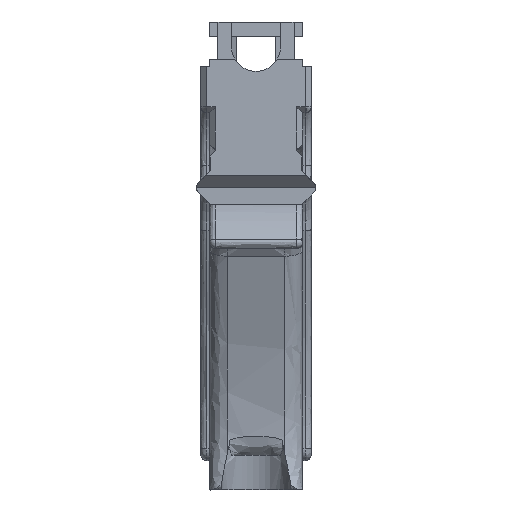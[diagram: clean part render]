
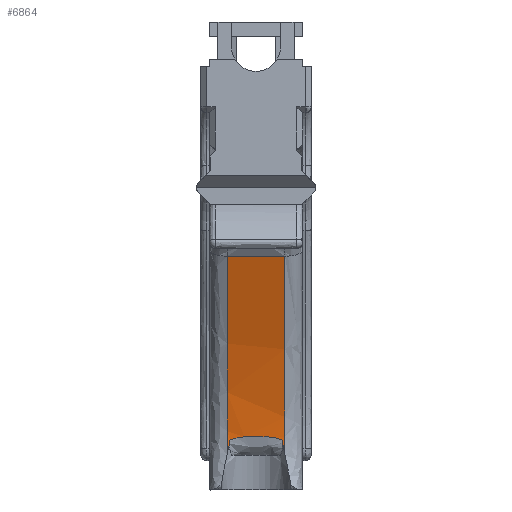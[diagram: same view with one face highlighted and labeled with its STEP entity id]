
A CAD part, front view. The second image highlights one B-rep face of the part: STEP entity #6864.
In plain terms, the highlighted free-form (B-spline) face has degree [5, 1] with [25, 2] control points.
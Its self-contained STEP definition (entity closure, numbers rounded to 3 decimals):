
#20=(
BOUNDED_SURFACE()
B_SPLINE_SURFACE(5,1,((#10581,#10582),(#10583,#10584),(#10585,#10586),(#10587,
#10588),(#10589,#10590),(#10591,#10592),(#10593,#10594),(#10595,#10596),
(#10597,#10598),(#10599,#10600),(#10601,#10602),(#10603,#10604),(#10605,
#10606),(#10607,#10608),(#10609,#10610),(#10611,#10612),(#10613,#10614),
(#10615,#10616),(#10617,#10618),(#10619,#10620),(#10621,#10622),(#10623,
#10624),(#10625,#10626),(#10627,#10628),(#10629,#10630)),.UNSPECIFIED.,
 .F.,.F.,.F.)
B_SPLINE_SURFACE_WITH_KNOTS((6,5,1,1,1,1,1,1,1,1,1,5,6),(2,2),(-1.404,
0.,0.1,0.2,0.3,0.4,0.5,0.6,0.7,0.8,0.9,1.,1.483),(-0.318,
1.908),.UNSPECIFIED.)
GEOMETRIC_REPRESENTATION_ITEM()
RATIONAL_B_SPLINE_SURFACE(((1.,1.),(1.,1.),(1.,1.),(1.,1.),(1.,1.),(1.,
1.),(1.,1.),(1.,1.),(1.,1.),(1.,1.),(1.,1.),(1.,1.),(1.,1.),(1.,1.),(1.,
1.),(1.,1.),(1.,1.),(1.,1.),(1.,1.),(1.,1.),(1.,1.),(1.,1.),(1.,1.),(1.,
1.),(1.,1.)))
REPRESENTATION_ITEM('')
SURFACE()
);
#200=B_SPLINE_CURVE_WITH_KNOTS('',3,(#10518,#10519,#10520,#10521,#10522,
#10523,#10524,#10525,#10526),.UNSPECIFIED.,.F.,.F.,(4,1,1,1,1,1,4),(-0.959,
-0.877,-0.755,-0.632,-0.386,
-0.141,-0.059),.UNSPECIFIED.);
#202=B_SPLINE_CURVE_WITH_KNOTS('',3,(#10632,#10633,#10634,#10635),
 .UNSPECIFIED.,.F.,.F.,(4,4),(-0.911,-0.711),
 .UNSPECIFIED.);
#203=B_SPLINE_CURVE_WITH_KNOTS('',3,(#10637,#10638,#10639,#10640,#10641,
#10642,#10643),.UNSPECIFIED.,.F.,.F.,(4,1,1,1,4),(-4.241,-2.995,
-1.749,-1.126,-0.582),.UNSPECIFIED.);
#204=B_SPLINE_CURVE_WITH_KNOTS('',3,(#10645,#10646,#10647,#10648),
 .UNSPECIFIED.,.F.,.F.,(4,4),(-1.29,-0.3),
 .UNSPECIFIED.);
#205=B_SPLINE_CURVE_WITH_KNOTS('',3,(#10650,#10651,#10652,#10653,#10654,
#10655,#10656),.UNSPECIFIED.,.F.,.F.,(4,1,1,1,4),(0.582,1.126,
1.749,2.995,4.241),.UNSPECIFIED.);
#206=B_SPLINE_CURVE_WITH_KNOTS('',3,(#10657,#10658,#10659,#10660),
 .UNSPECIFIED.,.F.,.F.,(4,4),(-0.243,0.),.UNSPECIFIED.);
#616=FACE_OUTER_BOUND('',#1000,.T.);
#1000=EDGE_LOOP('',(#4863,#4864,#4865,#4866,#4867,#4868));
#3012=VERTEX_POINT('',#10463);
#3014=VERTEX_POINT('',#10517);
#3016=VERTEX_POINT('',#10631);
#3017=VERTEX_POINT('',#10636);
#3018=VERTEX_POINT('',#10644);
#3019=VERTEX_POINT('',#10649);
#3720=EDGE_CURVE('',#3012,#3014,#200,.T.);
#3723=EDGE_CURVE('',#3016,#3012,#202,.T.);
#3724=EDGE_CURVE('',#3017,#3016,#203,.T.);
#3725=EDGE_CURVE('',#3018,#3017,#204,.T.);
#3726=EDGE_CURVE('',#3019,#3018,#205,.T.);
#3727=EDGE_CURVE('',#3014,#3019,#206,.T.);
#4863=ORIENTED_EDGE('',*,*,#3723,.F.);
#4864=ORIENTED_EDGE('',*,*,#3724,.F.);
#4865=ORIENTED_EDGE('',*,*,#3725,.F.);
#4866=ORIENTED_EDGE('',*,*,#3726,.F.);
#4867=ORIENTED_EDGE('',*,*,#3727,.F.);
#4868=ORIENTED_EDGE('',*,*,#3720,.F.);
#6864=ADVANCED_FACE('',(#616),#20,.F.);
#10463=CARTESIAN_POINT('',(12.379,-27.933,-61.535));
#10517=CARTESIAN_POINT('',(3.521,-27.933,-61.535));
#10518=CARTESIAN_POINT('Ctrl Pts',(12.379,-27.933,-61.535));
#10519=CARTESIAN_POINT('Ctrl Pts',(12.129,-27.934,-61.435));
#10520=CARTESIAN_POINT('Ctrl Pts',(11.484,-27.939,-61.226));
#10521=CARTESIAN_POINT('Ctrl Pts',(10.413,-27.946,-61.033));
#10522=CARTESIAN_POINT('Ctrl Pts',(8.771,-27.95,-60.907));
#10523=CARTESIAN_POINT('Ctrl Pts',(6.718,-27.951,-60.907));
#10524=CARTESIAN_POINT('Ctrl Pts',(4.803,-27.942,-61.102));
#10525=CARTESIAN_POINT('Ctrl Pts',(3.77,-27.934,-61.435));
#10526=CARTESIAN_POINT('Ctrl Pts',(3.521,-27.933,-61.535));
#10581=CARTESIAN_POINT('Ctrl Pts',(-3.18,-48.861,
-96.18));
#10582=CARTESIAN_POINT('Ctrl Pts',(19.08,-48.861,-96.18));
#10583=CARTESIAN_POINT('Ctrl Pts',(-3.18,-45.092,
-90.944));
#10584=CARTESIAN_POINT('Ctrl Pts',(19.08,-45.092,-90.944));
#10585=CARTESIAN_POINT('Ctrl Pts',(-3.18,-41.323,
-85.709));
#10586=CARTESIAN_POINT('Ctrl Pts',(19.08,-41.323,-85.709));
#10587=CARTESIAN_POINT('Ctrl Pts',(-3.18,-37.554,
-80.474));
#10588=CARTESIAN_POINT('Ctrl Pts',(19.08,-37.554,-80.474));
#10589=CARTESIAN_POINT('Ctrl Pts',(-3.18,-33.785,
-75.238));
#10590=CARTESIAN_POINT('Ctrl Pts',(19.08,-33.785,-75.238));
#10591=CARTESIAN_POINT('Ctrl Pts',(-3.18,-30.016,
-70.003));
#10592=CARTESIAN_POINT('Ctrl Pts',(19.08,-30.016,-70.003));
#10593=CARTESIAN_POINT('Ctrl Pts',(-3.18,-29.748,
-69.63));
#10594=CARTESIAN_POINT('Ctrl Pts',(19.08,-29.748,-69.63));
#10595=CARTESIAN_POINT('Ctrl Pts',(-3.18,-29.253,
-68.836));
#10596=CARTESIAN_POINT('Ctrl Pts',(19.08,-29.253,-68.836));
#10597=CARTESIAN_POINT('Ctrl Pts',(-3.18,-28.637,
-67.498));
#10598=CARTESIAN_POINT('Ctrl Pts',(19.08,-28.637,-67.498));
#10599=CARTESIAN_POINT('Ctrl Pts',(-3.18,-28.071,
-65.416));
#10600=CARTESIAN_POINT('Ctrl Pts',(19.08,-28.071,-65.416));
#10601=CARTESIAN_POINT('Ctrl Pts',(-3.18,-27.812,
-62.291));
#10602=CARTESIAN_POINT('Ctrl Pts',(19.08,-27.812,-62.291));
#10603=CARTESIAN_POINT('Ctrl Pts',(-3.18,-28.022,
-58.621));
#10604=CARTESIAN_POINT('Ctrl Pts',(19.08,-28.022,-58.621));
#10605=CARTESIAN_POINT('Ctrl Pts',(-3.18,-28.695,-54.412));
#10606=CARTESIAN_POINT('Ctrl Pts',(19.08,-28.695,-54.412));
#10607=CARTESIAN_POINT('Ctrl Pts',(-3.18,-29.793,
-49.709));
#10608=CARTESIAN_POINT('Ctrl Pts',(19.08,-29.793,-49.709));
#10609=CARTESIAN_POINT('Ctrl Pts',(-3.18,-31.267,
-44.567));
#10610=CARTESIAN_POINT('Ctrl Pts',(19.08,-31.267,-44.567));
#10611=CARTESIAN_POINT('Ctrl Pts',(-3.18,-33.073,
-39.04));
#10612=CARTESIAN_POINT('Ctrl Pts',(19.08,-33.073,-39.04));
#10613=CARTESIAN_POINT('Ctrl Pts',(-3.18,-34.754,
-34.343));
#10614=CARTESIAN_POINT('Ctrl Pts',(19.08,-34.754,-34.343));
#10615=CARTESIAN_POINT('Ctrl Pts',(-3.18,-36.138,
-30.676));
#10616=CARTESIAN_POINT('Ctrl Pts',(19.08,-36.138,-30.676));
#10617=CARTESIAN_POINT('Ctrl Pts',(-3.18,-37.114,
-28.169));
#10618=CARTESIAN_POINT('Ctrl Pts',(19.08,-37.114,-28.169));
#10619=CARTESIAN_POINT('Ctrl Pts',(-3.18,-37.616,
-26.9));
#10620=CARTESIAN_POINT('Ctrl Pts',(19.08,-37.616,-26.9));
#10621=CARTESIAN_POINT('Ctrl Pts',(-3.18,-40.039,
-20.77));
#10622=CARTESIAN_POINT('Ctrl Pts',(19.08,-40.039,-20.77));
#10623=CARTESIAN_POINT('Ctrl Pts',(-3.18,-42.463,
-14.639));
#10624=CARTESIAN_POINT('Ctrl Pts',(19.08,-42.463,-14.639));
#10625=CARTESIAN_POINT('Ctrl Pts',(-3.18,-44.886,
-8.508));
#10626=CARTESIAN_POINT('Ctrl Pts',(19.08,-44.886,-8.508));
#10627=CARTESIAN_POINT('Ctrl Pts',(-3.18,-47.31,
-2.377));
#10628=CARTESIAN_POINT('Ctrl Pts',(19.08,-47.31,-2.377));
#10629=CARTESIAN_POINT('Ctrl Pts',(-3.18,-49.733,
3.753));
#10630=CARTESIAN_POINT('Ctrl Pts',(19.08,-49.733,3.753));
#10631=CARTESIAN_POINT('',(12.9,-28.025,-64.081));
#10632=CARTESIAN_POINT('Ctrl Pts',(12.9,-28.025,-64.081));
#10633=CARTESIAN_POINT('Ctrl Pts',(12.725,-27.948,-63.278));
#10634=CARTESIAN_POINT('Ctrl Pts',(12.546,-27.917,-62.431));
#10635=CARTESIAN_POINT('Ctrl Pts',(12.379,-27.933,-61.535));
#10636=CARTESIAN_POINT('',(12.9,-36.357,-30.134));
#10637=CARTESIAN_POINT('Ctrl Pts',(12.9,-36.357,-30.134));
#10638=CARTESIAN_POINT('Ctrl Pts',(12.9,-34.885,-33.976));
#10639=CARTESIAN_POINT('Ctrl Pts',(12.9,-32.101,-41.691));
#10640=CARTESIAN_POINT('Ctrl Pts',(12.9,-29.234,-51.473));
#10641=CARTESIAN_POINT('Ctrl Pts',(12.9,-27.951,-59.002));
#10642=CARTESIAN_POINT('Ctrl Pts',(12.9,-27.874,-62.525));
#10643=CARTESIAN_POINT('Ctrl Pts',(12.9,-28.026,-64.08));
#10644=CARTESIAN_POINT('',(3.,-36.357,-30.134));
#10645=CARTESIAN_POINT('Ctrl Pts',(3.,-36.357,-30.134));
#10646=CARTESIAN_POINT('Ctrl Pts',(6.3,-36.357,-30.134));
#10647=CARTESIAN_POINT('Ctrl Pts',(9.6,-36.357,-30.134));
#10648=CARTESIAN_POINT('Ctrl Pts',(12.9,-36.357,-30.134));
#10649=CARTESIAN_POINT('',(3.,-28.025,-64.081));
#10650=CARTESIAN_POINT('Ctrl Pts',(3.,-28.025,-64.081));
#10651=CARTESIAN_POINT('Ctrl Pts',(3.,-27.873,-62.524));
#10652=CARTESIAN_POINT('Ctrl Pts',(3.,-27.952,-58.998));
#10653=CARTESIAN_POINT('Ctrl Pts',(3.,-29.234,-51.471));
#10654=CARTESIAN_POINT('Ctrl Pts',(3.,-32.102,-41.689));
#10655=CARTESIAN_POINT('Ctrl Pts',(3.,-34.885,-33.975));
#10656=CARTESIAN_POINT('Ctrl Pts',(3.,-36.357,-30.134));
#10657=CARTESIAN_POINT('Ctrl Pts',(3.521,-27.933,-61.535));
#10658=CARTESIAN_POINT('Ctrl Pts',(3.351,-27.917,-62.445));
#10659=CARTESIAN_POINT('Ctrl Pts',(3.172,-27.949,-63.291));
#10660=CARTESIAN_POINT('Ctrl Pts',(3.,-28.025,-64.081));
